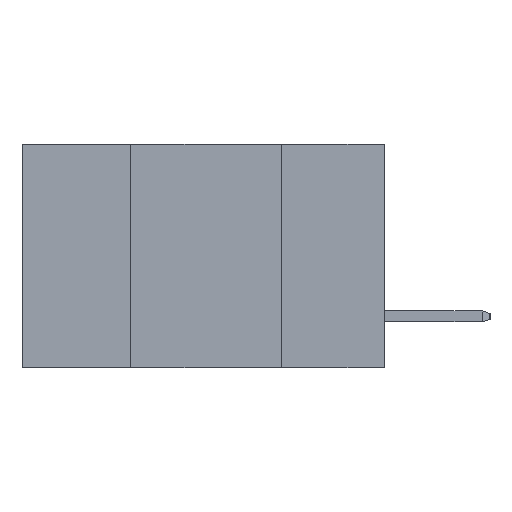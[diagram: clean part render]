
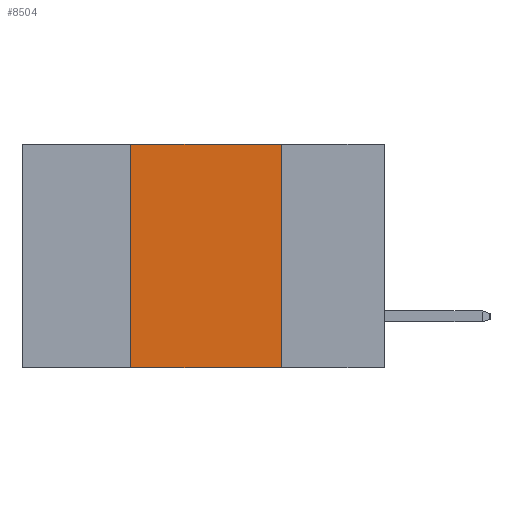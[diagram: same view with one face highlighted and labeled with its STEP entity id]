
A CAD part, left-side view. The second image highlights one B-rep face of the part: STEP entity #8504.
In plain terms, the highlighted planar face has unit normal (-1, 0, 0).
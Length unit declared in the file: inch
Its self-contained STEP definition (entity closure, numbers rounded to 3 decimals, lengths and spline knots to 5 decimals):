
#651 = CARTESIAN_POINT ( 'NONE',  ( 0., 0.17, -0.37 ) ) ;
#1157 = CARTESIAN_POINT ( 'NONE',  ( 0., 0.42, 0. ) ) ;
#1423 = DIRECTION ( 'NONE',  ( 0., -1., 0. ) ) ;
#1618 = EDGE_LOOP ( 'NONE', ( #7330, #2340, #8023, #3232 ) ) ;
#1746 = DIRECTION ( 'NONE',  ( 0., 0., -1. ) ) ;
#2055 = FACE_OUTER_BOUND ( 'NONE', #1618, .T. ) ;
#2340 = ORIENTED_EDGE ( 'NONE', *, *, #6839, .F. ) ;
#2366 = LINE ( 'NONE', #8838, #7604 ) ;
#2431 = VECTOR ( 'NONE', #1423, 39.37008 ) ;
#2510 = VECTOR ( 'NONE', #1746, 39.37008 ) ;
#3039 = DIRECTION ( 'NONE',  ( 1., 0., 0. ) ) ;
#3170 = VERTEX_POINT ( 'NONE', #8574 ) ;
#3232 = ORIENTED_EDGE ( 'NONE', *, *, #10984, .T. ) ;
#4049 = CARTESIAN_POINT ( 'NONE',  ( 0., 0.6, -0.37 ) ) ;
#4869 = VERTEX_POINT ( 'NONE', #6298 ) ;
#5181 = LINE ( 'NONE', #10716, #2431 ) ;
#5975 = VERTEX_POINT ( 'NONE', #11496 ) ;
#6298 = CARTESIAN_POINT ( 'NONE',  ( 0., 0.17, -0.37 ) ) ;
#6839 = EDGE_CURVE ( 'NONE', #9806, #3170, #5181, .T. ) ;
#7330 = ORIENTED_EDGE ( 'NONE', *, *, #9549, .F. ) ;
#7604 = VECTOR ( 'NONE', #7801, 39.37008 ) ;
#7801 = DIRECTION ( 'NONE',  ( 0., 0., 1. ) ) ;
#8023 = ORIENTED_EDGE ( 'NONE', *, *, #13159, .F. ) ;
#8504 = ADVANCED_FACE ( 'NONE', ( #2055 ), #9297, .F. ) ;
#8574 = CARTESIAN_POINT ( 'NONE',  ( 0., 0.17, 0. ) ) ;
#8632 = LINE ( 'NONE', #4049, #10715 ) ;
#8838 = CARTESIAN_POINT ( 'NONE',  ( 0., 0.42, -0.37 ) ) ;
#9259 = DIRECTION ( 'NONE',  ( 0., -1., 0. ) ) ;
#9297 = PLANE ( 'NONE',  #9803 ) ;
#9549 = EDGE_CURVE ( 'NONE', #3170, #4869, #13149, .T. ) ;
#9803 = AXIS2_PLACEMENT_3D ( 'NONE', #11294, #3039, #10315 ) ;
#9806 = VERTEX_POINT ( 'NONE', #1157 ) ;
#10315 = DIRECTION ( 'NONE',  ( 0., 0., -1. ) ) ;
#10715 = VECTOR ( 'NONE', #9259, 39.37008 ) ;
#10716 = CARTESIAN_POINT ( 'NONE',  ( 0., 0.6, 0. ) ) ;
#10984 = EDGE_CURVE ( 'NONE', #5975, #4869, #8632, .T. ) ;
#11294 = CARTESIAN_POINT ( 'NONE',  ( 0., 0.6, 0. ) ) ;
#11496 = CARTESIAN_POINT ( 'NONE',  ( 0., 0.42, -0.37 ) ) ;
#13149 = LINE ( 'NONE', #651, #2510 ) ;
#13159 = EDGE_CURVE ( 'NONE', #5975, #9806, #2366, .T. ) ;
